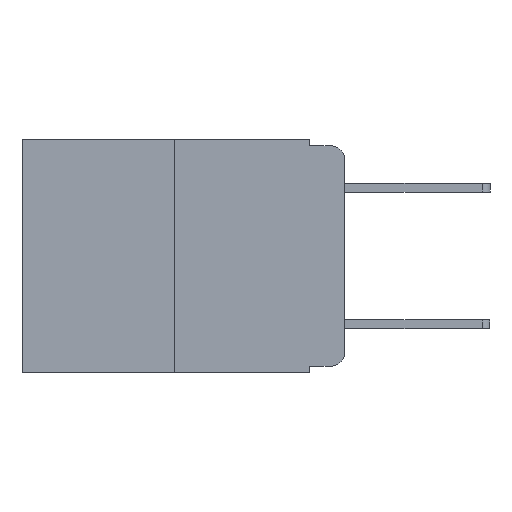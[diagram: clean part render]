
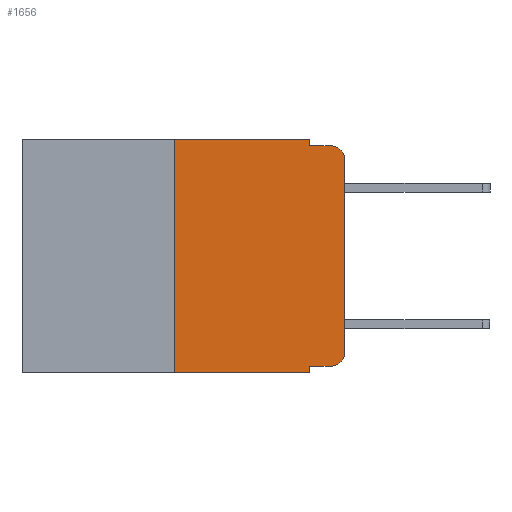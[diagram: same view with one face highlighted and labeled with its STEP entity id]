
A CAD part, left-side view. The second image highlights one B-rep face of the part: STEP entity #1656.
In plain terms, the highlighted planar face has unit normal (-1, 0, 0).
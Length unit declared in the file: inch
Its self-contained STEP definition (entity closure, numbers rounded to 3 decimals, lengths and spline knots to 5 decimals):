
#366 = ORIENTED_EDGE ( 'NONE', *, *, #2317, .F. ) ;
#533 = CARTESIAN_POINT ( 'NONE',  ( 0., 0.473, 0. ) ) ;
#658 = EDGE_CURVE ( 'NONE', #8590, #1442, #11430, .T. ) ;
#675 = VERTEX_POINT ( 'NONE', #8144 ) ;
#964 = ORIENTED_EDGE ( 'NONE', *, *, #5969, .T. ) ;
#1107 = EDGE_LOOP ( 'NONE', ( #7681, #1393, #18539, #14447, #6997, #9199, #2136, #366, #2782, #964 ) ) ;
#1146 = LINE ( 'NONE', #17604, #16129 ) ;
#1208 = DIRECTION ( 'NONE',  ( -1., 0., 0. ) ) ;
#1393 = ORIENTED_EDGE ( 'NONE', *, *, #658, .T. ) ;
#1442 = VERTEX_POINT ( 'NONE', #12089 ) ;
#1462 = AXIS2_PLACEMENT_3D ( 'NONE', #11643, #2677, #13113 ) ;
#1656 = ADVANCED_FACE ( 'NONE', ( #5657 ), #2525, .F. ) ;
#1845 = EDGE_CURVE ( 'NONE', #17266, #17124, #14114, .T. ) ;
#2136 = ORIENTED_EDGE ( 'NONE', *, *, #2698, .T. ) ;
#2184 = EDGE_CURVE ( 'NONE', #9341, #1442, #3661, .T. ) ;
#2317 = EDGE_CURVE ( 'NONE', #675, #16241, #1146, .T. ) ;
#2374 = CARTESIAN_POINT ( 'NONE',  ( 0., 0., -0.313 ) ) ;
#2525 = PLANE ( 'NONE',  #10948 ) ;
#2677 = DIRECTION ( 'NONE',  ( -1., 0., 0. ) ) ;
#2698 = EDGE_CURVE ( 'NONE', #13788, #16241, #11572, .T. ) ;
#2782 = ORIENTED_EDGE ( 'NONE', *, *, #16581, .T. ) ;
#3661 = LINE ( 'NONE', #7759, #6817 ) ;
#4322 = CARTESIAN_POINT ( 'NONE',  ( 0., 0.25, 0. ) ) ;
#4388 = DIRECTION ( 'NONE',  ( 0., 0., -1. ) ) ;
#4845 = CARTESIAN_POINT ( 'NONE',  ( 0., 0.051, -0.343 ) ) ;
#5203 = VECTOR ( 'NONE', #10601, 39.37008 ) ;
#5299 = DIRECTION ( 'NONE',  ( 0., 0., -1. ) ) ;
#5643 = CARTESIAN_POINT ( 'NONE',  ( 0., 0.25, -0.343 ) ) ;
#5657 = FACE_OUTER_BOUND ( 'NONE', #1107, .T. ) ;
#5895 = VECTOR ( 'NONE', #9202, 39.37008 ) ;
#5969 = EDGE_CURVE ( 'NONE', #12184, #16510, #8042, .T. ) ;
#6126 = EDGE_CURVE ( 'NONE', #13788, #17266, #11433, .T. ) ;
#6158 = LINE ( 'NONE', #9448, #9172 ) ;
#6203 = CARTESIAN_POINT ( 'NONE',  ( 0., 0., -0.03 ) ) ;
#6225 = EDGE_CURVE ( 'NONE', #16510, #8590, #11649, .T. ) ;
#6544 = CARTESIAN_POINT ( 'NONE',  ( 0., 0.02, -0.03 ) ) ;
#6817 = VECTOR ( 'NONE', #16874, 39.37008 ) ;
#6888 = LINE ( 'NONE', #7189, #14616 ) ;
#6997 = ORIENTED_EDGE ( 'NONE', *, *, #1845, .F. ) ;
#7189 = CARTESIAN_POINT ( 'NONE',  ( 0., 0.051, -0.333 ) ) ;
#7528 = CARTESIAN_POINT ( 'NONE',  ( 0., 0.02, -0.333 ) ) ;
#7681 = ORIENTED_EDGE ( 'NONE', *, *, #6225, .T. ) ;
#7759 = CARTESIAN_POINT ( 'NONE',  ( 0., 0.051, -0.01 ) ) ;
#7809 = VECTOR ( 'NONE', #10774, 39.37008 ) ;
#8042 = CIRCLE ( 'NONE', #1462, 0.02 ) ;
#8144 = CARTESIAN_POINT ( 'NONE',  ( 0., 0.051, -0.333 ) ) ;
#8307 = CARTESIAN_POINT ( 'NONE',  ( 0., 0.473, 0. ) ) ;
#8590 = VERTEX_POINT ( 'NONE', #6203 ) ;
#9145 = CARTESIAN_POINT ( 'NONE',  ( 0., 0.25, 0. ) ) ;
#9172 = VECTOR ( 'NONE', #10881, 39.37008 ) ;
#9199 = ORIENTED_EDGE ( 'NONE', *, *, #6126, .F. ) ;
#9202 = DIRECTION ( 'NONE',  ( 0., -1., 0. ) ) ;
#9341 = VERTEX_POINT ( 'NONE', #11058 ) ;
#9448 = CARTESIAN_POINT ( 'NONE',  ( 0., 0.051, 0. ) ) ;
#10601 = DIRECTION ( 'NONE',  ( 0., 0., 1. ) ) ;
#10686 = EDGE_CURVE ( 'NONE', #17124, #9341, #6158, .T. ) ;
#10774 = DIRECTION ( 'NONE',  ( 0., 0., 1. ) ) ;
#10881 = DIRECTION ( 'NONE',  ( 0., 0., -1. ) ) ;
#10948 = AXIS2_PLACEMENT_3D ( 'NONE', #8307, #16118, #16134 ) ;
#11058 = CARTESIAN_POINT ( 'NONE',  ( 0., 0.051, -0.01 ) ) ;
#11411 = CARTESIAN_POINT ( 'NONE',  ( 0., 0.051, 0. ) ) ;
#11430 = CIRCLE ( 'NONE', #15681, 0.02 ) ;
#11433 = LINE ( 'NONE', #9145, #5203 ) ;
#11572 = LINE ( 'NONE', #19072, #18706 ) ;
#11643 = CARTESIAN_POINT ( 'NONE',  ( 0., 0.02, -0.313 ) ) ;
#11649 = LINE ( 'NONE', #17898, #7809 ) ;
#12089 = CARTESIAN_POINT ( 'NONE',  ( 0., 0.02, -0.01 ) ) ;
#12184 = VERTEX_POINT ( 'NONE', #7528 ) ;
#13025 = DIRECTION ( 'NONE',  ( 0., -1., 0. ) ) ;
#13113 = DIRECTION ( 'NONE',  ( 0., 0., -1. ) ) ;
#13639 = DIRECTION ( 'NONE',  ( 0., -1., 0. ) ) ;
#13788 = VERTEX_POINT ( 'NONE', #5643 ) ;
#14114 = LINE ( 'NONE', #533, #5895 ) ;
#14447 = ORIENTED_EDGE ( 'NONE', *, *, #10686, .F. ) ;
#14616 = VECTOR ( 'NONE', #13025, 39.37008 ) ;
#15681 = AXIS2_PLACEMENT_3D ( 'NONE', #6544, #1208, #4388 ) ;
#16118 = DIRECTION ( 'NONE',  ( 1., 0., 0. ) ) ;
#16129 = VECTOR ( 'NONE', #5299, 39.37008 ) ;
#16134 = DIRECTION ( 'NONE',  ( 0., 0., -1. ) ) ;
#16241 = VERTEX_POINT ( 'NONE', #4845 ) ;
#16510 = VERTEX_POINT ( 'NONE', #2374 ) ;
#16581 = EDGE_CURVE ( 'NONE', #675, #12184, #6888, .T. ) ;
#16874 = DIRECTION ( 'NONE',  ( 0., -1., 0. ) ) ;
#17124 = VERTEX_POINT ( 'NONE', #11411 ) ;
#17266 = VERTEX_POINT ( 'NONE', #4322 ) ;
#17604 = CARTESIAN_POINT ( 'NONE',  ( 0., 0.051, 0. ) ) ;
#17898 = CARTESIAN_POINT ( 'NONE',  ( 0., 0., 0. ) ) ;
#18539 = ORIENTED_EDGE ( 'NONE', *, *, #2184, .F. ) ;
#18706 = VECTOR ( 'NONE', #13639, 39.37008 ) ;
#19072 = CARTESIAN_POINT ( 'NONE',  ( 0., 0.473, -0.343 ) ) ;
